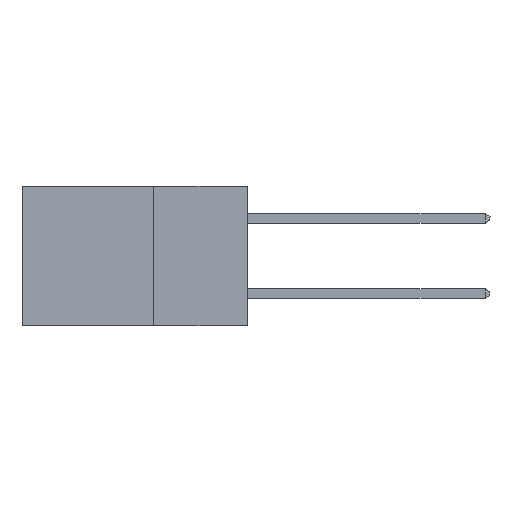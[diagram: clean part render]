
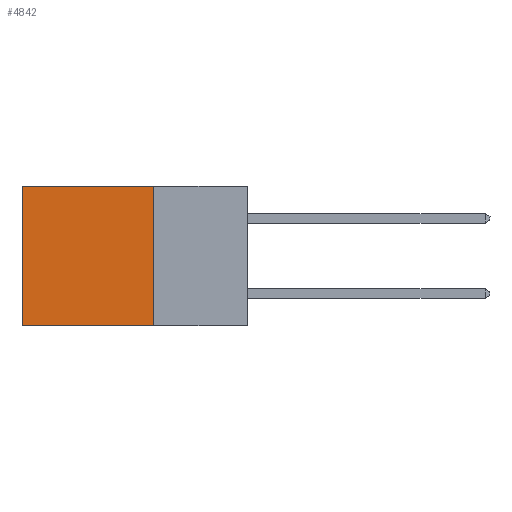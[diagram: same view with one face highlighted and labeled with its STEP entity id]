
A CAD part, left-side view. The second image highlights one B-rep face of the part: STEP entity #4842.
In plain terms, the highlighted planar face has unit normal (-1, 0, 0).
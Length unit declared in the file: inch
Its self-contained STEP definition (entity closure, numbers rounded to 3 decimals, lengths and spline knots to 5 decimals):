
#291 = CARTESIAN_POINT ( 'NONE',  ( 0.2615, 0.6, -0.37 ) ) ;
#483 = VERTEX_POINT ( 'NONE', #7203 ) ;
#595 = CARTESIAN_POINT ( 'NONE',  ( 0.2615, 0.25, 0. ) ) ;
#618 = DIRECTION ( 'NONE',  ( 0., 0., -1. ) ) ;
#731 = CARTESIAN_POINT ( 'NONE',  ( 0.2615, 0.6, -0.37 ) ) ;
#1105 = ORIENTED_EDGE ( 'NONE', *, *, #6314, .T. ) ;
#1403 = PLANE ( 'NONE',  #7395 ) ;
#1468 = VERTEX_POINT ( 'NONE', #3131 ) ;
#1562 = DIRECTION ( 'NONE',  ( 1., 0., 0. ) ) ;
#1588 = DIRECTION ( 'NONE',  ( 0., 1., 0. ) ) ;
#1622 = DIRECTION ( 'NONE',  ( 0., 0., -1. ) ) ;
#2114 = VERTEX_POINT ( 'NONE', #595 ) ;
#2382 = LINE ( 'NONE', #731, #8856 ) ;
#2395 = LINE ( 'NONE', #8581, #7543 ) ;
#2603 = CARTESIAN_POINT ( 'NONE',  ( 0.2615, 0.25, -0.37 ) ) ;
#2972 = CARTESIAN_POINT ( 'NONE',  ( 0.2615, 0.25, -0.37 ) ) ;
#3131 = CARTESIAN_POINT ( 'NONE',  ( 0.2615, 0.25, -0.37 ) ) ;
#3454 = LINE ( 'NONE', #2603, #9512 ) ;
#4128 = CARTESIAN_POINT ( 'NONE',  ( 0.2615, 0.25, -0.37 ) ) ;
#4842 = ADVANCED_FACE ( 'NONE', ( #5430 ), #1403, .F. ) ;
#5089 = DIRECTION ( 'NONE',  ( 0., 0., -1. ) ) ;
#5430 = FACE_OUTER_BOUND ( 'NONE', #5638, .T. ) ;
#5638 = EDGE_LOOP ( 'NONE', ( #1105, #5718, #9527, #5883 ) ) ;
#5718 = ORIENTED_EDGE ( 'NONE', *, *, #9253, .F. ) ;
#5801 = EDGE_CURVE ( 'NONE', #2114, #483, #2395, .T. ) ;
#5883 = ORIENTED_EDGE ( 'NONE', *, *, #5801, .T. ) ;
#6314 = EDGE_CURVE ( 'NONE', #483, #6967, #2382, .T. ) ;
#6954 = EDGE_CURVE ( 'NONE', #2114, #1468, #3454, .T. ) ;
#6967 = VERTEX_POINT ( 'NONE', #291 ) ;
#7203 = CARTESIAN_POINT ( 'NONE',  ( 0.2615, 0.6, 0. ) ) ;
#7253 = DIRECTION ( 'NONE',  ( 0., 1., 0. ) ) ;
#7395 = AXIS2_PLACEMENT_3D ( 'NONE', #2972, #1562, #618 ) ;
#7543 = VECTOR ( 'NONE', #1588, 39.37008 ) ;
#8075 = LINE ( 'NONE', #4128, #8584 ) ;
#8581 = CARTESIAN_POINT ( 'NONE',  ( 0.2615, 0.25, 0. ) ) ;
#8584 = VECTOR ( 'NONE', #7253, 39.37008 ) ;
#8856 = VECTOR ( 'NONE', #1622, 39.37008 ) ;
#9253 = EDGE_CURVE ( 'NONE', #1468, #6967, #8075, .T. ) ;
#9512 = VECTOR ( 'NONE', #5089, 39.37008 ) ;
#9527 = ORIENTED_EDGE ( 'NONE', *, *, #6954, .F. ) ;
